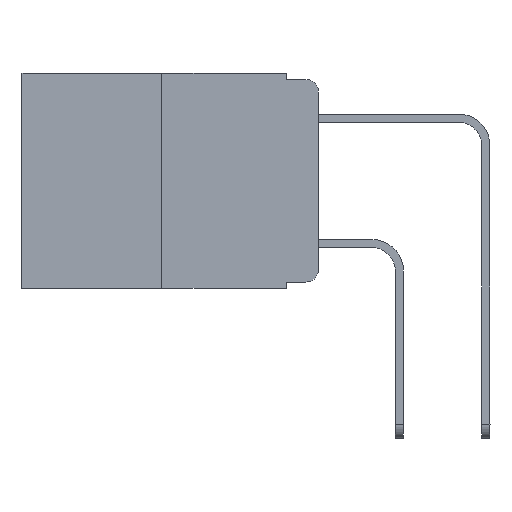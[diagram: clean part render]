
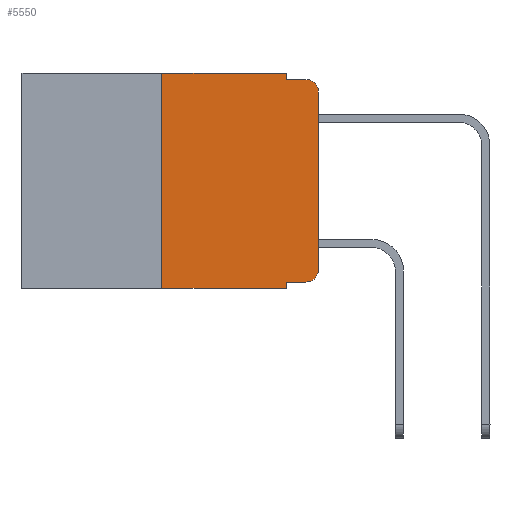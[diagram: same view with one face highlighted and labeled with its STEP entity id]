
A CAD part, left-side view. The second image highlights one B-rep face of the part: STEP entity #5550.
In plain terms, the highlighted planar face has unit normal (-1, 0, 0).
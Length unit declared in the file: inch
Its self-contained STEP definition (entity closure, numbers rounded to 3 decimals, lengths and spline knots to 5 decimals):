
#72 = VECTOR ( 'NONE', #5690, 39.37008 ) ;
#619 = EDGE_CURVE ( 'NONE', #3680, #4904, #1207, .T. ) ;
#687 = ORIENTED_EDGE ( 'NONE', *, *, #5366, .T. ) ;
#849 = AXIS2_PLACEMENT_3D ( 'NONE', #7070, #10665, #4352 ) ;
#850 = VERTEX_POINT ( 'NONE', #5345 ) ;
#921 = CARTESIAN_POINT ( 'NONE',  ( 0., 0.051, 0. ) ) ;
#1037 = DIRECTION ( 'NONE',  ( 0., 0., -1. ) ) ;
#1207 = LINE ( 'NONE', #9205, #6490 ) ;
#1299 = CARTESIAN_POINT ( 'NONE',  ( 0., 0.051, -0.333 ) ) ;
#1335 = LINE ( 'NONE', #6755, #7188 ) ;
#1593 = LINE ( 'NONE', #1704, #5178 ) ;
#1607 = CIRCLE ( 'NONE', #849, 0.02 ) ;
#1637 = ORIENTED_EDGE ( 'NONE', *, *, #2906, .F. ) ;
#1704 = CARTESIAN_POINT ( 'NONE',  ( 0., 0.473, 0. ) ) ;
#1743 = VERTEX_POINT ( 'NONE', #10621 ) ;
#1817 = DIRECTION ( 'NONE',  ( 0., -1., 0. ) ) ;
#1835 = CARTESIAN_POINT ( 'NONE',  ( 0., 0.051, -0.01 ) ) ;
#2026 = VERTEX_POINT ( 'NONE', #1835 ) ;
#2054 = DIRECTION ( 'NONE',  ( 0., 0., -1. ) ) ;
#2112 = AXIS2_PLACEMENT_3D ( 'NONE', #8284, #7283, #1037 ) ;
#2255 = VERTEX_POINT ( 'NONE', #4293 ) ;
#2373 = VECTOR ( 'NONE', #7751, 39.37008 ) ;
#2379 = LINE ( 'NONE', #9790, #2373 ) ;
#2806 = DIRECTION ( 'NONE',  ( -1., 0., 0. ) ) ;
#2906 = EDGE_CURVE ( 'NONE', #3442, #1743, #5806, .T. ) ;
#3000 = LINE ( 'NONE', #5666, #3648 ) ;
#3064 = CIRCLE ( 'NONE', #10025, 0.02 ) ;
#3442 = VERTEX_POINT ( 'NONE', #1299 ) ;
#3637 = ORIENTED_EDGE ( 'NONE', *, *, #7745, .T. ) ;
#3648 = VECTOR ( 'NONE', #5726, 39.37008 ) ;
#3678 = PLANE ( 'NONE',  #2112 ) ;
#3680 = VERTEX_POINT ( 'NONE', #10657 ) ;
#3816 = CARTESIAN_POINT ( 'NONE',  ( 0., 0., -0.313 ) ) ;
#3851 = CARTESIAN_POINT ( 'NONE',  ( 0., 0.02, -0.01 ) ) ;
#3975 = CARTESIAN_POINT ( 'NONE',  ( 0., 0., 0. ) ) ;
#3982 = VECTOR ( 'NONE', #7940, 39.37008 ) ;
#4025 = VECTOR ( 'NONE', #6278, 39.37008 ) ;
#4287 = VERTEX_POINT ( 'NONE', #3851 ) ;
#4293 = CARTESIAN_POINT ( 'NONE',  ( 0., 0., -0.03 ) ) ;
#4352 = DIRECTION ( 'NONE',  ( 0., 0., -1. ) ) ;
#4736 = DIRECTION ( 'NONE',  ( 0., 0., 1. ) ) ;
#4904 = VERTEX_POINT ( 'NONE', #6737 ) ;
#5036 = ORIENTED_EDGE ( 'NONE', *, *, #7168, .T. ) ;
#5178 = VECTOR ( 'NONE', #1817, 39.37008 ) ;
#5227 = CARTESIAN_POINT ( 'NONE',  ( 0., 0.473, -0.343 ) ) ;
#5345 = CARTESIAN_POINT ( 'NONE',  ( 0., 0.051, 0. ) ) ;
#5366 = EDGE_CURVE ( 'NONE', #3680, #1743, #9698, .T. ) ;
#5457 = FACE_OUTER_BOUND ( 'NONE', #8435, .T. ) ;
#5550 = ADVANCED_FACE ( 'NONE', ( #5457 ), #3678, .F. ) ;
#5615 = EDGE_CURVE ( 'NONE', #850, #2026, #1335, .T. ) ;
#5666 = CARTESIAN_POINT ( 'NONE',  ( 0., 0.051, -0.01 ) ) ;
#5690 = DIRECTION ( 'NONE',  ( 0., 0., 1. ) ) ;
#5726 = DIRECTION ( 'NONE',  ( 0., -1., 0. ) ) ;
#5806 = LINE ( 'NONE', #921, #4025 ) ;
#6146 = ORIENTED_EDGE ( 'NONE', *, *, #9903, .F. ) ;
#6278 = DIRECTION ( 'NONE',  ( 0., 0., -1. ) ) ;
#6490 = VECTOR ( 'NONE', #4736, 39.37008 ) ;
#6737 = CARTESIAN_POINT ( 'NONE',  ( 0., 0.25, 0. ) ) ;
#6755 = CARTESIAN_POINT ( 'NONE',  ( 0., 0.051, 0. ) ) ;
#7027 = CARTESIAN_POINT ( 'NONE',  ( 0., 0.02, -0.333 ) ) ;
#7034 = ORIENTED_EDGE ( 'NONE', *, *, #5615, .F. ) ;
#7070 = CARTESIAN_POINT ( 'NONE',  ( 0., 0.02, -0.03 ) ) ;
#7071 = ORIENTED_EDGE ( 'NONE', *, *, #8923, .T. ) ;
#7168 = EDGE_CURVE ( 'NONE', #8375, #10313, #3064, .T. ) ;
#7188 = VECTOR ( 'NONE', #11174, 39.37008 ) ;
#7283 = DIRECTION ( 'NONE',  ( 1., 0., 0. ) ) ;
#7745 = EDGE_CURVE ( 'NONE', #10313, #2255, #10284, .T. ) ;
#7751 = DIRECTION ( 'NONE',  ( 0., -1., 0. ) ) ;
#7940 = DIRECTION ( 'NONE',  ( 0., -1., 0. ) ) ;
#8284 = CARTESIAN_POINT ( 'NONE',  ( 0., 0.473, 0. ) ) ;
#8375 = VERTEX_POINT ( 'NONE', #7027 ) ;
#8435 = EDGE_LOOP ( 'NONE', ( #3637, #7071, #6146, #7034, #9874, #11488, #687, #1637, #11500, #5036 ) ) ;
#8849 = EDGE_CURVE ( 'NONE', #4904, #850, #1593, .T. ) ;
#8923 = EDGE_CURVE ( 'NONE', #2255, #4287, #1607, .T. ) ;
#9205 = CARTESIAN_POINT ( 'NONE',  ( 0., 0.25, 0. ) ) ;
#9612 = EDGE_CURVE ( 'NONE', #3442, #8375, #2379, .T. ) ;
#9698 = LINE ( 'NONE', #5227, #3982 ) ;
#9790 = CARTESIAN_POINT ( 'NONE',  ( 0., 0.051, -0.333 ) ) ;
#9874 = ORIENTED_EDGE ( 'NONE', *, *, #8849, .F. ) ;
#9903 = EDGE_CURVE ( 'NONE', #2026, #4287, #3000, .T. ) ;
#10025 = AXIS2_PLACEMENT_3D ( 'NONE', #11012, #2806, #2054 ) ;
#10284 = LINE ( 'NONE', #3975, #72 ) ;
#10313 = VERTEX_POINT ( 'NONE', #3816 ) ;
#10621 = CARTESIAN_POINT ( 'NONE',  ( 0., 0.051, -0.343 ) ) ;
#10657 = CARTESIAN_POINT ( 'NONE',  ( 0., 0.25, -0.343 ) ) ;
#10665 = DIRECTION ( 'NONE',  ( -1., 0., 0. ) ) ;
#11012 = CARTESIAN_POINT ( 'NONE',  ( 0., 0.02, -0.313 ) ) ;
#11174 = DIRECTION ( 'NONE',  ( 0., 0., -1. ) ) ;
#11488 = ORIENTED_EDGE ( 'NONE', *, *, #619, .F. ) ;
#11500 = ORIENTED_EDGE ( 'NONE', *, *, #9612, .T. ) ;
